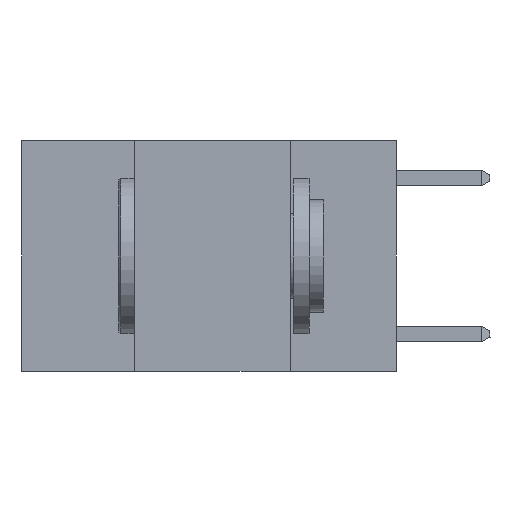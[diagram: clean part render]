
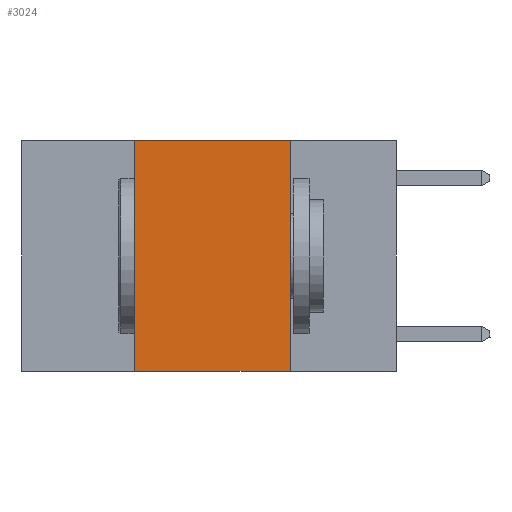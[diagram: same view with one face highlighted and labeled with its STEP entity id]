
A CAD part, left-side view. The second image highlights one B-rep face of the part: STEP entity #3024.
In plain terms, the highlighted planar face has unit normal (-1, 0, 0).
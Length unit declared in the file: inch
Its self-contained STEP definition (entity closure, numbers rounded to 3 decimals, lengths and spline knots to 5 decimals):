
#494 = LINE ( 'NONE', #8465, #9008 ) ;
#1068 = CARTESIAN_POINT ( 'NONE',  ( 0., 0.17, 0. ) ) ;
#1135 = VECTOR ( 'NONE', #6801, 39.37008 ) ;
#1313 = VERTEX_POINT ( 'NONE', #10965 ) ;
#1388 = AXIS2_PLACEMENT_3D ( 'NONE', #5988, #7266, #15482 ) ;
#2108 = VERTEX_POINT ( 'NONE', #1068 ) ;
#2352 = ORIENTED_EDGE ( 'NONE', *, *, #8364, .F. ) ;
#3024 = ADVANCED_FACE ( 'NONE', ( #7559 ), #10558, .F. ) ;
#3621 = CARTESIAN_POINT ( 'NONE',  ( 0., 0.6, -0.37 ) ) ;
#4118 = EDGE_CURVE ( 'NONE', #8658, #1313, #7175, .T. ) ;
#4571 = CARTESIAN_POINT ( 'NONE',  ( 0., 0.42, 0. ) ) ;
#5632 = ORIENTED_EDGE ( 'NONE', *, *, #8615, .F. ) ;
#5988 = CARTESIAN_POINT ( 'NONE',  ( 0., 0.6, 0. ) ) ;
#6801 = DIRECTION ( 'NONE',  ( 0., 0., -1. ) ) ;
#7138 = VECTOR ( 'NONE', #10993, 39.37008 ) ;
#7175 = LINE ( 'NONE', #3621, #17534 ) ;
#7266 = DIRECTION ( 'NONE',  ( 1., 0., 0. ) ) ;
#7559 = FACE_OUTER_BOUND ( 'NONE', #12104, .T. ) ;
#8127 = CARTESIAN_POINT ( 'NONE',  ( 0., 0.17, 0. ) ) ;
#8350 = ORIENTED_EDGE ( 'NONE', *, *, #4118, .T. ) ;
#8364 = EDGE_CURVE ( 'NONE', #2108, #1313, #11441, .T. ) ;
#8429 = CARTESIAN_POINT ( 'NONE',  ( 0., 0.42, 0. ) ) ;
#8465 = CARTESIAN_POINT ( 'NONE',  ( 0., 0.6, 0. ) ) ;
#8615 = EDGE_CURVE ( 'NONE', #8658, #19743, #13704, .T. ) ;
#8658 = VERTEX_POINT ( 'NONE', #17743 ) ;
#9008 = VECTOR ( 'NONE', #16468, 39.37008 ) ;
#10558 = PLANE ( 'NONE',  #1388 ) ;
#10965 = CARTESIAN_POINT ( 'NONE',  ( 0., 0.17, -0.37 ) ) ;
#10993 = DIRECTION ( 'NONE',  ( 0., 0., 1. ) ) ;
#11441 = LINE ( 'NONE', #8127, #1135 ) ;
#12104 = EDGE_LOOP ( 'NONE', ( #2352, #12793, #5632, #8350 ) ) ;
#12793 = ORIENTED_EDGE ( 'NONE', *, *, #14519, .F. ) ;
#13704 = LINE ( 'NONE', #4571, #7138 ) ;
#14519 = EDGE_CURVE ( 'NONE', #19743, #2108, #494, .T. ) ;
#15482 = DIRECTION ( 'NONE',  ( 0., 0., -1. ) ) ;
#16468 = DIRECTION ( 'NONE',  ( 0., -1., 0. ) ) ;
#17534 = VECTOR ( 'NONE', #17831, 39.37008 ) ;
#17743 = CARTESIAN_POINT ( 'NONE',  ( 0., 0.42, -0.37 ) ) ;
#17831 = DIRECTION ( 'NONE',  ( 0., -1., 0. ) ) ;
#19743 = VERTEX_POINT ( 'NONE', #8429 ) ;
